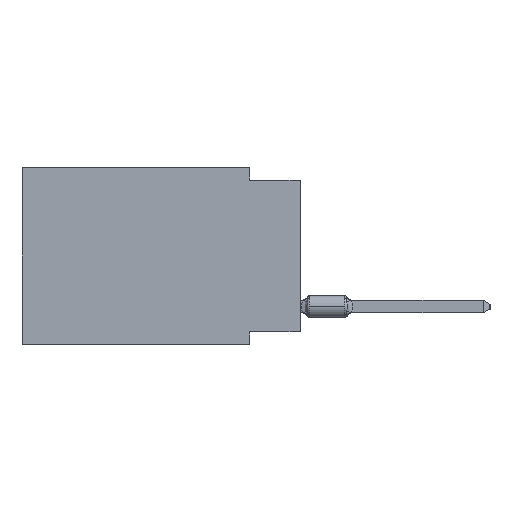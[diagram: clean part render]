
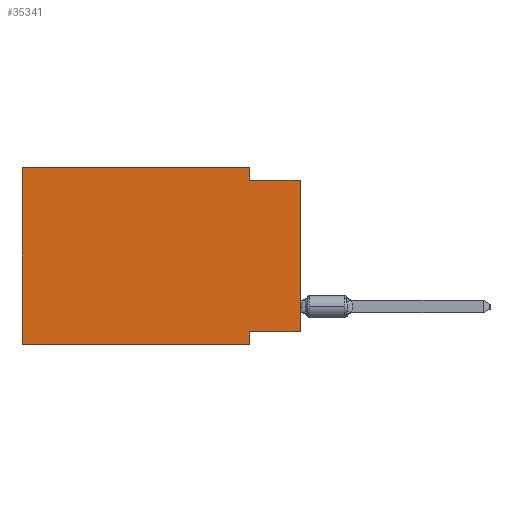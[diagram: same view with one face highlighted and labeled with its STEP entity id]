
A CAD part, left-side view. The second image highlights one B-rep face of the part: STEP entity #35341.
In plain terms, the highlighted planar face has unit normal (-1, 0, 0).
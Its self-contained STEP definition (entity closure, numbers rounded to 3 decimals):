
#609 = LINE ( 'NONE', #12560, #81166 ) ;
#692 = VERTEX_POINT ( 'NONE', #19552 ) ;
#1035 = EDGE_CURVE ( 'NONE', #72204, #52775, #43351, .T. ) ;
#1321 = EDGE_CURVE ( 'NONE', #23444, #81410, #72518, .T. ) ;
#2645 = ORIENTED_EDGE ( 'NONE', *, *, #1321, .F. ) ;
#3233 = CARTESIAN_POINT ( 'NONE',  ( 0., 13.97, 0. ) ) ;
#3576 = LINE ( 'NONE', #10556, #20504 ) ;
#3822 = CARTESIAN_POINT ( 'NONE',  ( 0., 13.97, 0. ) ) ;
#6942 = DIRECTION ( 'NONE',  ( 0., 0., 1. ) ) ;
#7743 = CARTESIAN_POINT ( 'NONE',  ( 0., 2.54, 0. ) ) ;
#9293 = EDGE_LOOP ( 'NONE', ( #20347, #40722, #19324, #27665, #2645, #42970, #32080, #42190 ) ) ;
#10556 = CARTESIAN_POINT ( 'NONE',  ( 0., 13.97, 0. ) ) ;
#12560 = CARTESIAN_POINT ( 'NONE',  ( 0., 2.54, 0. ) ) ;
#13160 = DIRECTION ( 'NONE',  ( 0., -1., 0. ) ) ;
#16809 = DIRECTION ( 'NONE',  ( 1., 0., 0. ) ) ;
#17405 = CARTESIAN_POINT ( 'NONE',  ( 0., 13.97, -8.89 ) ) ;
#18282 = CARTESIAN_POINT ( 'NONE',  ( 0., 0., -8.255 ) ) ;
#19324 = ORIENTED_EDGE ( 'NONE', *, *, #59696, .F. ) ;
#19347 = LINE ( 'NONE', #44439, #40016 ) ;
#19552 = CARTESIAN_POINT ( 'NONE',  ( 0., 0., -0.635 ) ) ;
#20080 = CARTESIAN_POINT ( 'NONE',  ( 0., 0., -0.635 ) ) ;
#20347 = ORIENTED_EDGE ( 'NONE', *, *, #49658, .T. ) ;
#20504 = VECTOR ( 'NONE', #72333, 1000. ) ;
#23444 = VERTEX_POINT ( 'NONE', #17405 ) ;
#23922 = AXIS2_PLACEMENT_3D ( 'NONE', #3233, #16809, #48083 ) ;
#25705 = VECTOR ( 'NONE', #41411, 1000. ) ;
#27665 = ORIENTED_EDGE ( 'NONE', *, *, #70367, .F. ) ;
#30940 = CARTESIAN_POINT ( 'NONE',  ( 0., 2.54, -8.89 ) ) ;
#32080 = ORIENTED_EDGE ( 'NONE', *, *, #41423, .F. ) ;
#33206 = EDGE_CURVE ( 'NONE', #23444, #75935, #19347, .T. ) ;
#33353 = VECTOR ( 'NONE', #6942, 1000. ) ;
#35341 = ADVANCED_FACE ( 'NONE', ( #73188 ), #71586, .F. ) ;
#37117 = DIRECTION ( 'NONE',  ( 0., 0., -1. ) ) ;
#38372 = CARTESIAN_POINT ( 'NONE',  ( 0., 0., -8.255 ) ) ;
#40016 = VECTOR ( 'NONE', #13160, 1000. ) ;
#40722 = ORIENTED_EDGE ( 'NONE', *, *, #69628, .F. ) ;
#40999 = CARTESIAN_POINT ( 'NONE',  ( 0., 2.54, -0.635 ) ) ;
#41411 = DIRECTION ( 'NONE',  ( 0., -1., 0. ) ) ;
#41423 = EDGE_CURVE ( 'NONE', #52775, #75935, #50280, .T. ) ;
#42190 = ORIENTED_EDGE ( 'NONE', *, *, #1035, .F. ) ;
#42970 = ORIENTED_EDGE ( 'NONE', *, *, #33206, .T. ) ;
#43351 = LINE ( 'NONE', #38372, #58918 ) ;
#44439 = CARTESIAN_POINT ( 'NONE',  ( 0., 13.97, -8.89 ) ) ;
#47007 = CARTESIAN_POINT ( 'NONE',  ( 0., 13.97, 0. ) ) ;
#48083 = DIRECTION ( 'NONE',  ( 0., 0., -1. ) ) ;
#49658 = EDGE_CURVE ( 'NONE', #72204, #692, #80295, .T. ) ;
#49768 = CARTESIAN_POINT ( 'NONE',  ( 0., 0., 0. ) ) ;
#50280 = LINE ( 'NONE', #30940, #60193 ) ;
#50820 = VERTEX_POINT ( 'NONE', #7743 ) ;
#52775 = VERTEX_POINT ( 'NONE', #55202 ) ;
#55202 = CARTESIAN_POINT ( 'NONE',  ( 0., 2.54, -8.255 ) ) ;
#58918 = VECTOR ( 'NONE', #62663, 1000. ) ;
#59696 = EDGE_CURVE ( 'NONE', #50820, #62536, #609, .T. ) ;
#60193 = VECTOR ( 'NONE', #37117, 1000. ) ;
#62536 = VERTEX_POINT ( 'NONE', #40999 ) ;
#62663 = DIRECTION ( 'NONE',  ( 0., 1., 0. ) ) ;
#63685 = LINE ( 'NONE', #20080, #25705 ) ;
#69367 = DIRECTION ( 'NONE',  ( 0., 0., -1. ) ) ;
#69628 = EDGE_CURVE ( 'NONE', #62536, #692, #63685, .T. ) ;
#70367 = EDGE_CURVE ( 'NONE', #81410, #50820, #3576, .T. ) ;
#71586 = PLANE ( 'NONE',  #23922 ) ;
#72114 = DIRECTION ( 'NONE',  ( 0., 0., 1. ) ) ;
#72204 = VERTEX_POINT ( 'NONE', #18282 ) ;
#72333 = DIRECTION ( 'NONE',  ( 0., -1., 0. ) ) ;
#72518 = LINE ( 'NONE', #47007, #73500 ) ;
#73188 = FACE_OUTER_BOUND ( 'NONE', #9293, .T. ) ;
#73500 = VECTOR ( 'NONE', #72114, 1000. ) ;
#75636 = CARTESIAN_POINT ( 'NONE',  ( 0., 2.54, -8.89 ) ) ;
#75935 = VERTEX_POINT ( 'NONE', #75636 ) ;
#80295 = LINE ( 'NONE', #49768, #33353 ) ;
#81166 = VECTOR ( 'NONE', #69367, 1000. ) ;
#81410 = VERTEX_POINT ( 'NONE', #3822 ) ;
